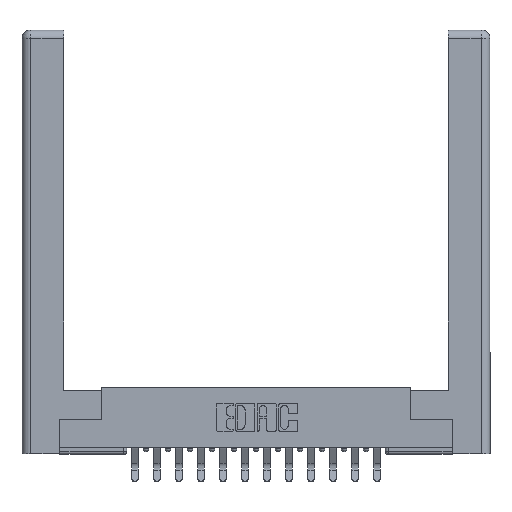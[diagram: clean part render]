
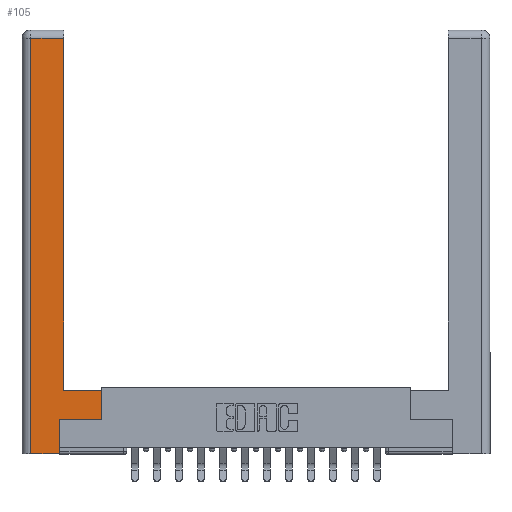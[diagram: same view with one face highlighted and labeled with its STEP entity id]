
A CAD part, top view. The second image highlights one B-rep face of the part: STEP entity #105.
In plain terms, the highlighted planar face has unit normal (0, 0, 1).
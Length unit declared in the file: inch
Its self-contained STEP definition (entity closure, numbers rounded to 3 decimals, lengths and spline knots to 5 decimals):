
#105 = ADVANCED_FACE ( 'NONE', ( #10426 ), #2575, .F. ) ;
#107 = ORIENTED_EDGE ( 'NONE', *, *, #15927, .T. ) ;
#1216 = VERTEX_POINT ( 'NONE', #9598 ) ;
#1590 = DIRECTION ( 'NONE',  ( 0., 1., 0. ) ) ;
#1713 = CARTESIAN_POINT ( 'NONE',  ( 0.295, 2.94, 0. ) ) ;
#1740 = CARTESIAN_POINT ( 'NONE',  ( 0.565, 0.245, 0. ) ) ;
#1938 = AXIS2_PLACEMENT_3D ( 'NONE', #15700, #3795, #9123 ) ;
#2563 = CARTESIAN_POINT ( 'NONE',  ( 0.265, 0., 0. ) ) ;
#2575 = PLANE ( 'NONE',  #1938 ) ;
#2691 = DIRECTION ( 'NONE',  ( -1., 0., 0. ) ) ;
#2771 = LINE ( 'NONE', #13870, #8278 ) ;
#2944 = ORIENTED_EDGE ( 'NONE', *, *, #6880, .T. ) ;
#3029 = ORIENTED_EDGE ( 'NONE', *, *, #6559, .T. ) ;
#3034 = EDGE_CURVE ( 'NONE', #6138, #1216, #9557, .T. ) ;
#3294 = VERTEX_POINT ( 'NONE', #1740 ) ;
#3438 = VECTOR ( 'NONE', #8354, 39.37008 ) ;
#3440 = CARTESIAN_POINT ( 'NONE',  ( 0.0615, 2.94, 0. ) ) ;
#3525 = DIRECTION ( 'NONE',  ( 0., 1., 0. ) ) ;
#3645 = DIRECTION ( 'NONE',  ( 1., 0., 0. ) ) ;
#3731 = LINE ( 'NONE', #4955, #4938 ) ;
#3795 = DIRECTION ( 'NONE',  ( 0., 0., -1. ) ) ;
#4240 = CARTESIAN_POINT ( 'NONE',  ( 0.295, 0.45, 0. ) ) ;
#4606 = CARTESIAN_POINT ( 'NONE',  ( 0.565, 0.45, 0. ) ) ;
#4938 = VECTOR ( 'NONE', #3645, 39.37008 ) ;
#4955 = CARTESIAN_POINT ( 'NONE',  ( 0.565, 0.245, 0. ) ) ;
#5209 = VERTEX_POINT ( 'NONE', #11101 ) ;
#5470 = VECTOR ( 'NONE', #9787, 39.37008 ) ;
#6138 = VERTEX_POINT ( 'NONE', #4606 ) ;
#6559 = EDGE_CURVE ( 'NONE', #13723, #15619, #2771, .T. ) ;
#6880 = EDGE_CURVE ( 'NONE', #15619, #9063, #12124, .T. ) ;
#6971 = CARTESIAN_POINT ( 'NONE',  ( 0.0615, 0., 0. ) ) ;
#6973 = CARTESIAN_POINT ( 'NONE',  ( 0.265, 0., 0. ) ) ;
#7724 = EDGE_CURVE ( 'NONE', #5209, #3294, #3731, .T. ) ;
#8252 = LINE ( 'NONE', #11016, #16246 ) ;
#8278 = VECTOR ( 'NONE', #2691, 39.37008 ) ;
#8354 = DIRECTION ( 'NONE',  ( -1., 0., 0. ) ) ;
#9063 = VERTEX_POINT ( 'NONE', #6971 ) ;
#9123 = DIRECTION ( 'NONE',  ( -1., 0., 0. ) ) ;
#9256 = LINE ( 'NONE', #14532, #15649 ) ;
#9557 = LINE ( 'NONE', #4240, #3438 ) ;
#9598 = CARTESIAN_POINT ( 'NONE',  ( 0.295, 0.45, 0. ) ) ;
#9787 = DIRECTION ( 'NONE',  ( 0., -1., 0. ) ) ;
#9824 = ORIENTED_EDGE ( 'NONE', *, *, #14456, .T. ) ;
#10149 = DIRECTION ( 'NONE',  ( 1., 0., 0. ) ) ;
#10426 = FACE_OUTER_BOUND ( 'NONE', #15660, .T. ) ;
#10470 = VECTOR ( 'NONE', #3525, 39.37008 ) ;
#11016 = CARTESIAN_POINT ( 'NONE',  ( 0.265, 0.245, 0. ) ) ;
#11101 = CARTESIAN_POINT ( 'NONE',  ( 0.265, 0.245, 0. ) ) ;
#12124 = LINE ( 'NONE', #12375, #5470 ) ;
#12375 = CARTESIAN_POINT ( 'NONE',  ( 0.0615, 0., 0. ) ) ;
#12507 = ORIENTED_EDGE ( 'NONE', *, *, #17048, .T. ) ;
#12596 = EDGE_CURVE ( 'NONE', #9063, #16557, #13168, .T. ) ;
#13079 = ORIENTED_EDGE ( 'NONE', *, *, #7724, .T. ) ;
#13168 = LINE ( 'NONE', #2563, #13911 ) ;
#13723 = VERTEX_POINT ( 'NONE', #1713 ) ;
#13870 = CARTESIAN_POINT ( 'NONE',  ( 0.0615, 2.94, 0. ) ) ;
#13911 = VECTOR ( 'NONE', #10149, 39.37008 ) ;
#14456 = EDGE_CURVE ( 'NONE', #3294, #6138, #9256, .T. ) ;
#14532 = CARTESIAN_POINT ( 'NONE',  ( 0.565, 0.45, 0. ) ) ;
#14617 = ORIENTED_EDGE ( 'NONE', *, *, #3034, .T. ) ;
#15098 = ORIENTED_EDGE ( 'NONE', *, *, #12596, .T. ) ;
#15178 = LINE ( 'NONE', #15427, #10470 ) ;
#15427 = CARTESIAN_POINT ( 'NONE',  ( 0.295, 3., 0. ) ) ;
#15619 = VERTEX_POINT ( 'NONE', #3440 ) ;
#15649 = VECTOR ( 'NONE', #16012, 39.37008 ) ;
#15660 = EDGE_LOOP ( 'NONE', ( #12507, #3029, #2944, #15098, #107, #13079, #9824, #14617 ) ) ;
#15700 = CARTESIAN_POINT ( 'NONE',  ( 0., 0., 0. ) ) ;
#15927 = EDGE_CURVE ( 'NONE', #16557, #5209, #8252, .T. ) ;
#16012 = DIRECTION ( 'NONE',  ( 0., 1., 0. ) ) ;
#16246 = VECTOR ( 'NONE', #1590, 39.37008 ) ;
#16557 = VERTEX_POINT ( 'NONE', #6973 ) ;
#17048 = EDGE_CURVE ( 'NONE', #1216, #13723, #15178, .T. ) ;
